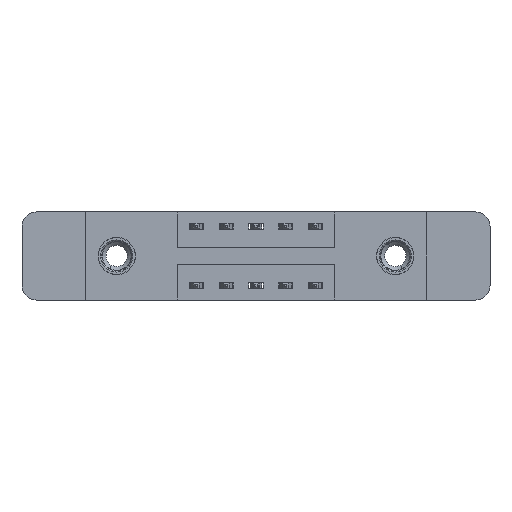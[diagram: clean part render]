
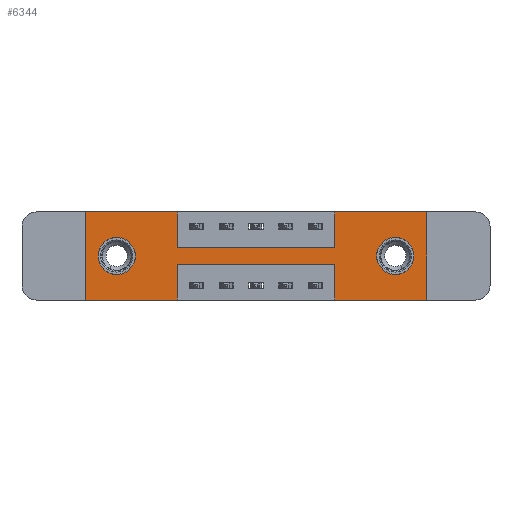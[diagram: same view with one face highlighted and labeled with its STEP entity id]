
A CAD part, front view. The second image highlights one B-rep face of the part: STEP entity #6344.
In plain terms, the highlighted planar face has unit normal (0, -1, 0).
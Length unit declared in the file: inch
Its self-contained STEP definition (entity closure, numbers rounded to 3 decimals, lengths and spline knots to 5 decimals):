
#59 = CARTESIAN_POINT ( 'NONE',  ( 0.3875, 0., 0. ) ) ;
#128 = EDGE_CURVE ( 'NONE', #1140, #9885, #12797, .T. ) ;
#131 = VECTOR ( 'NONE', #8543, 39.37008 ) ;
#214 = AXIS2_PLACEMENT_3D ( 'NONE', #1951, #9297, #12606 ) ;
#222 = VERTEX_POINT ( 'NONE', #11222 ) ;
#407 = VECTOR ( 'NONE', #2049, 39.37008 ) ;
#667 = VECTOR ( 'NONE', #4057, 39.37008 ) ;
#725 = FACE_BOUND ( 'NONE', #9035, .T. ) ;
#756 = CARTESIAN_POINT ( 'NONE',  ( 0., 0., -0.37 ) ) ;
#773 = CARTESIAN_POINT ( 'NONE',  ( 0., 0., 0. ) ) ;
#793 = EDGE_CURVE ( 'NONE', #4355, #3494, #5294, .T. ) ;
#809 = DIRECTION ( 'NONE',  ( 0., 0., 1. ) ) ;
#857 = VERTEX_POINT ( 'NONE', #6213 ) ;
#946 = DIRECTION ( 'NONE',  ( -1., 0., 0. ) ) ;
#1041 = LINE ( 'NONE', #773, #407 ) ;
#1140 = VERTEX_POINT ( 'NONE', #59 ) ;
#1145 = LINE ( 'NONE', #4289, #6411 ) ;
#1232 = LINE ( 'NONE', #12880, #5779 ) ;
#1273 = DIRECTION ( 'NONE',  ( 0., 1., 0. ) ) ;
#1448 = EDGE_LOOP ( 'NONE', ( #2273, #10381, #11077, #3592, #8780, #11134, #4596, #7067, #9174, #13350, #7109, #8477 ) ) ;
#1582 = CIRCLE ( 'NONE', #214, 0.078 ) ;
#1787 = FACE_BOUND ( 'NONE', #13807, .T. ) ;
#1951 = CARTESIAN_POINT ( 'NONE',  ( 1.3025, 0., -0.185 ) ) ;
#2049 = DIRECTION ( 'NONE',  ( 0., 0., 1. ) ) ;
#2177 = VERTEX_POINT ( 'NONE', #4678 ) ;
#2273 = ORIENTED_EDGE ( 'NONE', *, *, #2390, .F. ) ;
#2332 = VERTEX_POINT ( 'NONE', #7133 ) ;
#2353 = ORIENTED_EDGE ( 'NONE', *, *, #9179, .T. ) ;
#2381 = LINE ( 'NONE', #7668, #7372 ) ;
#2390 = EDGE_CURVE ( 'NONE', #2177, #4355, #1232, .T. ) ;
#2547 = DIRECTION ( 'NONE',  ( 0., 0., 1. ) ) ;
#2672 = VECTOR ( 'NONE', #809, 39.37008 ) ;
#2698 = VECTOR ( 'NONE', #4076, 39.37008 ) ;
#2856 = CARTESIAN_POINT ( 'NONE',  ( 1.3025, 0., -0.107 ) ) ;
#2860 = LINE ( 'NONE', #4174, #13199 ) ;
#2915 = CARTESIAN_POINT ( 'NONE',  ( 0., 0., 0. ) ) ;
#2985 = LINE ( 'NONE', #13650, #6503 ) ;
#2995 = EDGE_CURVE ( 'NONE', #3494, #11685, #1041, .T. ) ;
#3017 = VERTEX_POINT ( 'NONE', #5325 ) ;
#3113 = CARTESIAN_POINT ( 'NONE',  ( 0.1325, 0., -0.107 ) ) ;
#3289 = EDGE_CURVE ( 'NONE', #9885, #2332, #2381, .T. ) ;
#3427 = EDGE_CURVE ( 'NONE', #11685, #1140, #2860, .T. ) ;
#3494 = VERTEX_POINT ( 'NONE', #756 ) ;
#3592 = ORIENTED_EDGE ( 'NONE', *, *, #9190, .F. ) ;
#3847 = VERTEX_POINT ( 'NONE', #5935 ) ;
#4035 = DIRECTION ( 'NONE',  ( 0., 0., 1. ) ) ;
#4057 = DIRECTION ( 'NONE',  ( 0., 0., -1. ) ) ;
#4058 = VERTEX_POINT ( 'NONE', #3113 ) ;
#4076 = DIRECTION ( 'NONE',  ( 0., 0., 1. ) ) ;
#4173 = DIRECTION ( 'NONE',  ( 0., 0., -1. ) ) ;
#4174 = CARTESIAN_POINT ( 'NONE',  ( 0., 0., 0. ) ) ;
#4289 = CARTESIAN_POINT ( 'NONE',  ( 0.3875, 0., -0.22 ) ) ;
#4355 = VERTEX_POINT ( 'NONE', #9130 ) ;
#4370 = CARTESIAN_POINT ( 'NONE',  ( 1.3025, 0., -0.263 ) ) ;
#4412 = ORIENTED_EDGE ( 'NONE', *, *, #8807, .T. ) ;
#4572 = EDGE_CURVE ( 'NONE', #3017, #2177, #1145, .T. ) ;
#4596 = ORIENTED_EDGE ( 'NONE', *, *, #10310, .F. ) ;
#4678 = CARTESIAN_POINT ( 'NONE',  ( 0.3875, 0., -0.22 ) ) ;
#4692 = EDGE_CURVE ( 'NONE', #8403, #4058, #5544, .T. ) ;
#4946 = DIRECTION ( 'NONE',  ( 0., 1., 0. ) ) ;
#4967 = LINE ( 'NONE', #9238, #667 ) ;
#4987 = CARTESIAN_POINT ( 'NONE',  ( 1.0475, 0., -0.37 ) ) ;
#5042 = VERTEX_POINT ( 'NONE', #11144 ) ;
#5088 = VECTOR ( 'NONE', #6464, 39.37008 ) ;
#5164 = CARTESIAN_POINT ( 'NONE',  ( 1.0475, 0., 0. ) ) ;
#5175 = DIRECTION ( 'NONE',  ( 0., 1., 0. ) ) ;
#5210 = DIRECTION ( 'NONE',  ( -1., 0., 0. ) ) ;
#5294 = LINE ( 'NONE', #12815, #131 ) ;
#5325 = CARTESIAN_POINT ( 'NONE',  ( 1.0475, 0., -0.22 ) ) ;
#5521 = VERTEX_POINT ( 'NONE', #2856 ) ;
#5544 = CIRCLE ( 'NONE', #11577, 0.078 ) ;
#5779 = VECTOR ( 'NONE', #10701, 39.37008 ) ;
#5799 = EDGE_CURVE ( 'NONE', #857, #222, #8257, .T. ) ;
#5935 = CARTESIAN_POINT ( 'NONE',  ( 1.435, 0., -0.37 ) ) ;
#6213 = CARTESIAN_POINT ( 'NONE',  ( 1.0475, 0., 0. ) ) ;
#6344 = ADVANCED_FACE ( 'NONE', ( #725, #1787, #12297 ), #12228, .T. ) ;
#6411 = VECTOR ( 'NONE', #5210, 39.37008 ) ;
#6464 = DIRECTION ( 'NONE',  ( 0., 0., -1. ) ) ;
#6493 = CIRCLE ( 'NONE', #11185, 0.078 ) ;
#6503 = VECTOR ( 'NONE', #946, 39.37008 ) ;
#6661 = EDGE_CURVE ( 'NONE', #222, #3847, #4967, .T. ) ;
#6751 = LINE ( 'NONE', #4987, #2698 ) ;
#6889 = DIRECTION ( 'NONE',  ( 0., 0., -1. ) ) ;
#6911 = DIRECTION ( 'NONE',  ( 1., 0., 0. ) ) ;
#7067 = ORIENTED_EDGE ( 'NONE', *, *, #3289, .F. ) ;
#7109 = ORIENTED_EDGE ( 'NONE', *, *, #2995, .F. ) ;
#7133 = CARTESIAN_POINT ( 'NONE',  ( 1.0475, 0., -0.15 ) ) ;
#7138 = DIRECTION ( 'NONE',  ( 1., 0., 0. ) ) ;
#7372 = VECTOR ( 'NONE', #9799, 39.37008 ) ;
#7377 = VECTOR ( 'NONE', #6911, 39.37008 ) ;
#7443 = CARTESIAN_POINT ( 'NONE',  ( 1.3025, 0., -0.185 ) ) ;
#7668 = CARTESIAN_POINT ( 'NONE',  ( 0.3875, 0., -0.15 ) ) ;
#8257 = LINE ( 'NONE', #2915, #7377 ) ;
#8403 = VERTEX_POINT ( 'NONE', #10160 ) ;
#8477 = ORIENTED_EDGE ( 'NONE', *, *, #793, .F. ) ;
#8543 = DIRECTION ( 'NONE',  ( -1., 0., 0. ) ) ;
#8780 = ORIENTED_EDGE ( 'NONE', *, *, #6661, .F. ) ;
#8807 = EDGE_CURVE ( 'NONE', #9396, #5521, #6493, .T. ) ;
#8820 = EDGE_CURVE ( 'NONE', #5521, #9396, #1582, .T. ) ;
#9035 = EDGE_LOOP ( 'NONE', ( #9077, #4412 ) ) ;
#9077 = ORIENTED_EDGE ( 'NONE', *, *, #8820, .T. ) ;
#9130 = CARTESIAN_POINT ( 'NONE',  ( 0.3875, 0., -0.37 ) ) ;
#9172 = CIRCLE ( 'NONE', #10305, 0.078 ) ;
#9174 = ORIENTED_EDGE ( 'NONE', *, *, #128, .F. ) ;
#9179 = EDGE_CURVE ( 'NONE', #4058, #8403, #9172, .T. ) ;
#9190 = EDGE_CURVE ( 'NONE', #3847, #5042, #2985, .T. ) ;
#9238 = CARTESIAN_POINT ( 'NONE',  ( 1.435, 0., 0. ) ) ;
#9297 = DIRECTION ( 'NONE',  ( 0., 1., 0. ) ) ;
#9396 = VERTEX_POINT ( 'NONE', #4370 ) ;
#9799 = DIRECTION ( 'NONE',  ( 1., 0., 0. ) ) ;
#9885 = VERTEX_POINT ( 'NONE', #12284 ) ;
#10160 = CARTESIAN_POINT ( 'NONE',  ( 0.1325, 0., -0.263 ) ) ;
#10269 = ORIENTED_EDGE ( 'NONE', *, *, #4692, .T. ) ;
#10305 = AXIS2_PLACEMENT_3D ( 'NONE', #12724, #4946, #4035 ) ;
#10310 = EDGE_CURVE ( 'NONE', #2332, #857, #10414, .T. ) ;
#10313 = CARTESIAN_POINT ( 'NONE',  ( 0., 0., 0. ) ) ;
#10381 = ORIENTED_EDGE ( 'NONE', *, *, #4572, .F. ) ;
#10414 = LINE ( 'NONE', #5164, #2672 ) ;
#10515 = AXIS2_PLACEMENT_3D ( 'NONE', #11166, #13559, #6889 ) ;
#10701 = DIRECTION ( 'NONE',  ( 0., 0., -1. ) ) ;
#11077 = ORIENTED_EDGE ( 'NONE', *, *, #12378, .F. ) ;
#11134 = ORIENTED_EDGE ( 'NONE', *, *, #5799, .F. ) ;
#11144 = CARTESIAN_POINT ( 'NONE',  ( 1.0475, 0., -0.37 ) ) ;
#11166 = CARTESIAN_POINT ( 'NONE',  ( 0., 0., -0.37 ) ) ;
#11185 = AXIS2_PLACEMENT_3D ( 'NONE', #7443, #5175, #4173 ) ;
#11222 = CARTESIAN_POINT ( 'NONE',  ( 1.435, 0., 0. ) ) ;
#11577 = AXIS2_PLACEMENT_3D ( 'NONE', #12160, #1273, #2547 ) ;
#11685 = VERTEX_POINT ( 'NONE', #10313 ) ;
#11796 = CARTESIAN_POINT ( 'NONE',  ( 0.3875, 0., 0. ) ) ;
#12160 = CARTESIAN_POINT ( 'NONE',  ( 0.1325, 0., -0.185 ) ) ;
#12228 = PLANE ( 'NONE',  #10515 ) ;
#12284 = CARTESIAN_POINT ( 'NONE',  ( 0.3875, 0., -0.15 ) ) ;
#12297 = FACE_OUTER_BOUND ( 'NONE', #1448, .T. ) ;
#12378 = EDGE_CURVE ( 'NONE', #5042, #3017, #6751, .T. ) ;
#12606 = DIRECTION ( 'NONE',  ( 0., 0., -1. ) ) ;
#12724 = CARTESIAN_POINT ( 'NONE',  ( 0.1325, 0., -0.185 ) ) ;
#12797 = LINE ( 'NONE', #11796, #5088 ) ;
#12815 = CARTESIAN_POINT ( 'NONE',  ( 0., 0., -0.37 ) ) ;
#12880 = CARTESIAN_POINT ( 'NONE',  ( 0.3875, 0., -0.37 ) ) ;
#13199 = VECTOR ( 'NONE', #7138, 39.37008 ) ;
#13350 = ORIENTED_EDGE ( 'NONE', *, *, #3427, .F. ) ;
#13559 = DIRECTION ( 'NONE',  ( 0., -1., 0. ) ) ;
#13650 = CARTESIAN_POINT ( 'NONE',  ( 0., 0., -0.37 ) ) ;
#13807 = EDGE_LOOP ( 'NONE', ( #2353, #10269 ) ) ;
